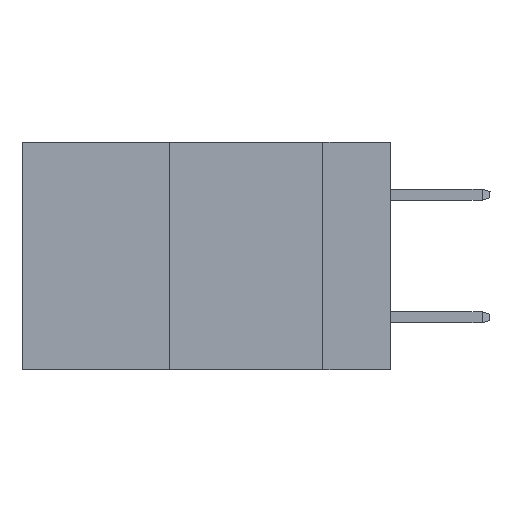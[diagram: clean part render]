
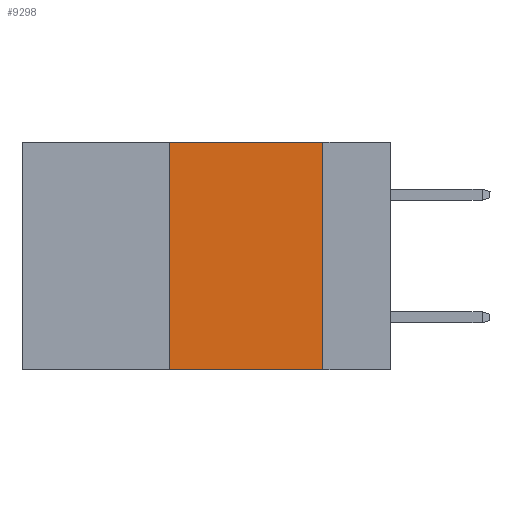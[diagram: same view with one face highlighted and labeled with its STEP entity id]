
A CAD part, left-side view. The second image highlights one B-rep face of the part: STEP entity #9298.
In plain terms, the highlighted planar face has unit normal (-1, 0, 0).
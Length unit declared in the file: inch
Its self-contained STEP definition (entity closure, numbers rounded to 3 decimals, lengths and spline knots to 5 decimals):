
#213 = VERTEX_POINT ( 'NONE', #4349 ) ;
#905 = VECTOR ( 'NONE', #3909, 39.37008 ) ;
#1243 = VECTOR ( 'NONE', #2834, 39.37008 ) ;
#1650 = CARTESIAN_POINT ( 'NONE',  ( 0., 0.11, 0. ) ) ;
#1670 = VECTOR ( 'NONE', #2409, 39.37008 ) ;
#2184 = DIRECTION ( 'NONE',  ( 1., 0., 0. ) ) ;
#2207 = EDGE_CURVE ( 'NONE', #3173, #8865, #5977, .T. ) ;
#2220 = EDGE_CURVE ( 'NONE', #213, #2285, #3036, .T. ) ;
#2285 = VERTEX_POINT ( 'NONE', #3185 ) ;
#2409 = DIRECTION ( 'NONE',  ( 0., 0., 1. ) ) ;
#2720 = EDGE_LOOP ( 'NONE', ( #7467, #2956, #3197, #5979 ) ) ;
#2834 = DIRECTION ( 'NONE',  ( 0., -1., 0. ) ) ;
#2956 = ORIENTED_EDGE ( 'NONE', *, *, #8296, .F. ) ;
#2995 = CARTESIAN_POINT ( 'NONE',  ( 0., 0.6, 0. ) ) ;
#3036 = LINE ( 'NONE', #8933, #1670 ) ;
#3173 = VERTEX_POINT ( 'NONE', #4075 ) ;
#3185 = CARTESIAN_POINT ( 'NONE',  ( 0., 0.36, 0. ) ) ;
#3197 = ORIENTED_EDGE ( 'NONE', *, *, #2220, .F. ) ;
#3623 = FACE_OUTER_BOUND ( 'NONE', #2720, .T. ) ;
#3909 = DIRECTION ( 'NONE',  ( 0., 0., -1. ) ) ;
#4075 = CARTESIAN_POINT ( 'NONE',  ( 0., 0.11, 0. ) ) ;
#4349 = CARTESIAN_POINT ( 'NONE',  ( 0., 0.36, -0.37 ) ) ;
#4391 = LINE ( 'NONE', #2995, #1243 ) ;
#5388 = VECTOR ( 'NONE', #6817, 39.37008 ) ;
#5859 = AXIS2_PLACEMENT_3D ( 'NONE', #6556, #2184, #6461 ) ;
#5977 = LINE ( 'NONE', #1650, #905 ) ;
#5979 = ORIENTED_EDGE ( 'NONE', *, *, #7913, .T. ) ;
#6461 = DIRECTION ( 'NONE',  ( 0., 0., -1. ) ) ;
#6556 = CARTESIAN_POINT ( 'NONE',  ( 0., 0.6, 0. ) ) ;
#6817 = DIRECTION ( 'NONE',  ( 0., -1., 0. ) ) ;
#7467 = ORIENTED_EDGE ( 'NONE', *, *, #2207, .F. ) ;
#7541 = LINE ( 'NONE', #9098, #5388 ) ;
#7913 = EDGE_CURVE ( 'NONE', #213, #8865, #7541, .T. ) ;
#8296 = EDGE_CURVE ( 'NONE', #2285, #3173, #4391, .T. ) ;
#8740 = PLANE ( 'NONE',  #5859 ) ;
#8865 = VERTEX_POINT ( 'NONE', #9254 ) ;
#8933 = CARTESIAN_POINT ( 'NONE',  ( 0., 0.36, 0. ) ) ;
#9098 = CARTESIAN_POINT ( 'NONE',  ( 0., 0.6, -0.37 ) ) ;
#9254 = CARTESIAN_POINT ( 'NONE',  ( 0., 0.11, -0.37 ) ) ;
#9298 = ADVANCED_FACE ( 'NONE', ( #3623 ), #8740, .F. ) ;
